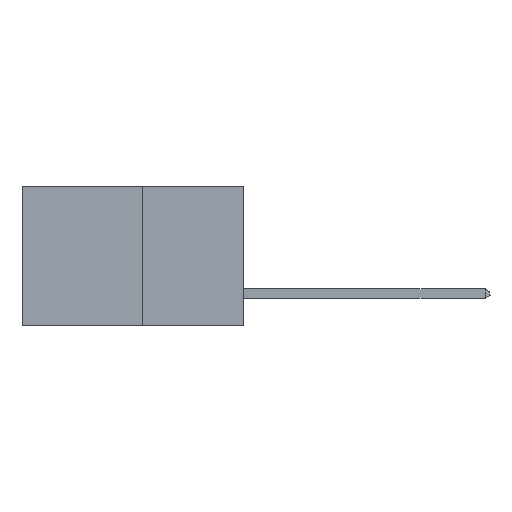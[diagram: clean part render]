
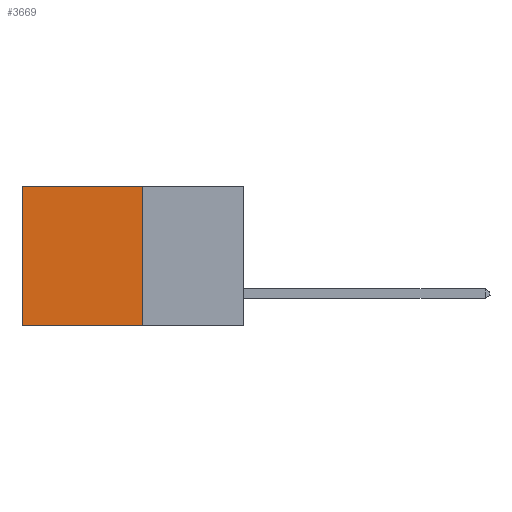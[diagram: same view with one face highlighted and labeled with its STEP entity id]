
A CAD part, left-side view. The second image highlights one B-rep face of the part: STEP entity #3669.
In plain terms, the highlighted planar face has unit normal (-1, 0, 0).
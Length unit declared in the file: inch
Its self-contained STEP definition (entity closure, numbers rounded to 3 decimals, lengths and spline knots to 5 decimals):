
#502 = ORIENTED_EDGE ( 'NONE', *, *, #1872, .T. ) ;
#653 = ORIENTED_EDGE ( 'NONE', *, *, #11468, .F. ) ;
#683 = LINE ( 'NONE', #5585, #9206 ) ;
#809 = ORIENTED_EDGE ( 'NONE', *, *, #5034, .F. ) ;
#939 = ORIENTED_EDGE ( 'NONE', *, *, #14295, .T. ) ;
#1286 = DIRECTION ( 'NONE',  ( 0., 0., -1. ) ) ;
#1574 = DIRECTION ( 'NONE',  ( 0., 0., -1. ) ) ;
#1872 = EDGE_CURVE ( 'NONE', #2200, #3550, #2163, .T. ) ;
#2163 = LINE ( 'NONE', #5791, #10890 ) ;
#2200 = VERTEX_POINT ( 'NONE', #12982 ) ;
#2451 = EDGE_LOOP ( 'NONE', ( #502, #653, #809, #939 ) ) ;
#3550 = VERTEX_POINT ( 'NONE', #13435 ) ;
#3669 = ADVANCED_FACE ( 'NONE', ( #5436 ), #11266, .F. ) ;
#3763 = VERTEX_POINT ( 'NONE', #12699 ) ;
#4163 = AXIS2_PLACEMENT_3D ( 'NONE', #7737, #7705, #1286 ) ;
#5034 = EDGE_CURVE ( 'NONE', #3763, #13560, #10990, .T. ) ;
#5436 = FACE_OUTER_BOUND ( 'NONE', #2451, .T. ) ;
#5585 = CARTESIAN_POINT ( 'NONE',  ( 0.277, 0.27, -0.37 ) ) ;
#5791 = CARTESIAN_POINT ( 'NONE',  ( 0.277, 0.59, -0.37 ) ) ;
#7705 = DIRECTION ( 'NONE',  ( 1., 0., 0. ) ) ;
#7737 = CARTESIAN_POINT ( 'NONE',  ( 0.277, 0.27, -0.37 ) ) ;
#8462 = CARTESIAN_POINT ( 'NONE',  ( 0.277, 0.27, -0.37 ) ) ;
#9206 = VECTOR ( 'NONE', #12163, 39.37008 ) ;
#9220 = CARTESIAN_POINT ( 'NONE',  ( 0.277, 0.27, 0. ) ) ;
#9291 = LINE ( 'NONE', #9220, #11766 ) ;
#9306 = DIRECTION ( 'NONE',  ( 0., 0., -1. ) ) ;
#9733 = CARTESIAN_POINT ( 'NONE',  ( 0.277, 0.27, -0.37 ) ) ;
#10323 = DIRECTION ( 'NONE',  ( 0., 1., 0. ) ) ;
#10653 = VECTOR ( 'NONE', #9306, 39.37008 ) ;
#10890 = VECTOR ( 'NONE', #1574, 39.37008 ) ;
#10990 = LINE ( 'NONE', #9733, #10653 ) ;
#11266 = PLANE ( 'NONE',  #4163 ) ;
#11468 = EDGE_CURVE ( 'NONE', #13560, #3550, #683, .T. ) ;
#11766 = VECTOR ( 'NONE', #10323, 39.37008 ) ;
#12163 = DIRECTION ( 'NONE',  ( 0., 1., 0. ) ) ;
#12699 = CARTESIAN_POINT ( 'NONE',  ( 0.277, 0.27, 0. ) ) ;
#12982 = CARTESIAN_POINT ( 'NONE',  ( 0.277, 0.59, 0. ) ) ;
#13435 = CARTESIAN_POINT ( 'NONE',  ( 0.277, 0.59, -0.37 ) ) ;
#13560 = VERTEX_POINT ( 'NONE', #8462 ) ;
#14295 = EDGE_CURVE ( 'NONE', #3763, #2200, #9291, .T. ) ;
